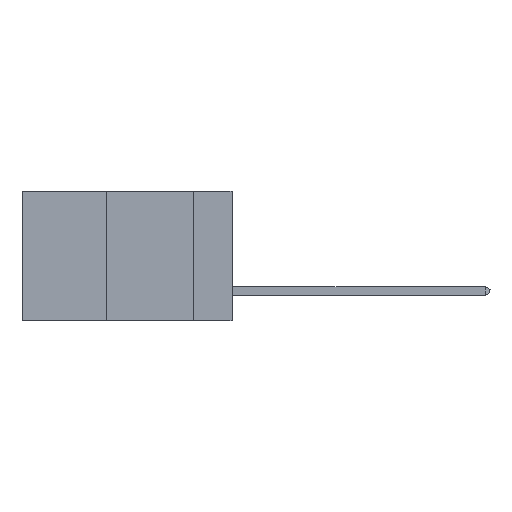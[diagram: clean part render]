
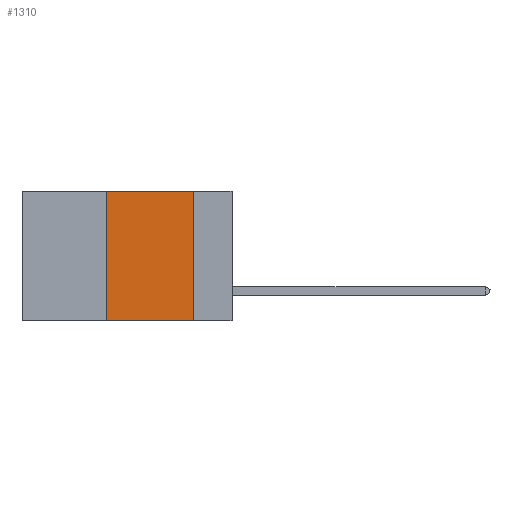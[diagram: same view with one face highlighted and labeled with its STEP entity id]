
A CAD part, left-side view. The second image highlights one B-rep face of the part: STEP entity #1310.
In plain terms, the highlighted planar face has unit normal (-1, 0, 0).
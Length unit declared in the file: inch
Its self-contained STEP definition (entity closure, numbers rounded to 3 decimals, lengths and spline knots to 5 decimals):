
#838 = ORIENTED_EDGE ( 'NONE', *, *, #8787, .F. ) ;
#1310 = ADVANCED_FACE ( 'NONE', ( #13364 ), #34710, .F. ) ;
#1548 = VECTOR ( 'NONE', #7268, 39.37008 ) ;
#2226 = DIRECTION ( 'NONE',  ( 0., 0., -1. ) ) ;
#2724 = ORIENTED_EDGE ( 'NONE', *, *, #13543, .F. ) ;
#6055 = EDGE_CURVE ( 'NONE', #22700, #18004, #16288, .T. ) ;
#7268 = DIRECTION ( 'NONE',  ( 0., 0., 1. ) ) ;
#8787 = EDGE_CURVE ( 'NONE', #15498, #22700, #21053, .T. ) ;
#9929 = CARTESIAN_POINT ( 'NONE',  ( 0., 0.36, 0. ) ) ;
#10812 = VECTOR ( 'NONE', #12277, 39.37008 ) ;
#11477 = ORIENTED_EDGE ( 'NONE', *, *, #6055, .F. ) ;
#11545 = CARTESIAN_POINT ( 'NONE',  ( 0., 0.11, 0. ) ) ;
#11572 = CARTESIAN_POINT ( 'NONE',  ( 0., 0.11, -0.37 ) ) ;
#12277 = DIRECTION ( 'NONE',  ( 0., -1., 0. ) ) ;
#13058 = EDGE_CURVE ( 'NONE', #13411, #18004, #17868, .T. ) ;
#13364 = FACE_OUTER_BOUND ( 'NONE', #16948, .T. ) ;
#13411 = VERTEX_POINT ( 'NONE', #15397 ) ;
#13543 = EDGE_CURVE ( 'NONE', #13411, #15498, #41147, .T. ) ;
#15269 = DIRECTION ( 'NONE',  ( 0., 0., -1. ) ) ;
#15397 = CARTESIAN_POINT ( 'NONE',  ( 0., 0.36, -0.37 ) ) ;
#15498 = VERTEX_POINT ( 'NONE', #9929 ) ;
#16288 = LINE ( 'NONE', #11545, #22893 ) ;
#16948 = EDGE_LOOP ( 'NONE', ( #11477, #838, #2724, #37770 ) ) ;
#17868 = LINE ( 'NONE', #36186, #40135 ) ;
#18004 = VERTEX_POINT ( 'NONE', #11572 ) ;
#21053 = LINE ( 'NONE', #32386, #10812 ) ;
#22700 = VERTEX_POINT ( 'NONE', #23381 ) ;
#22893 = VECTOR ( 'NONE', #15269, 39.37008 ) ;
#23381 = CARTESIAN_POINT ( 'NONE',  ( 0., 0.11, 0. ) ) ;
#23920 = DIRECTION ( 'NONE',  ( 0., -1., 0. ) ) ;
#25184 = DIRECTION ( 'NONE',  ( 1., 0., 0. ) ) ;
#29550 = CARTESIAN_POINT ( 'NONE',  ( 0., 0.36, 0. ) ) ;
#32386 = CARTESIAN_POINT ( 'NONE',  ( 0., 0.6, 0. ) ) ;
#34710 = PLANE ( 'NONE',  #41684 ) ;
#36186 = CARTESIAN_POINT ( 'NONE',  ( 0., 0.6, -0.37 ) ) ;
#37770 = ORIENTED_EDGE ( 'NONE', *, *, #13058, .T. ) ;
#38151 = CARTESIAN_POINT ( 'NONE',  ( 0., 0.6, 0. ) ) ;
#40135 = VECTOR ( 'NONE', #23920, 39.37008 ) ;
#41147 = LINE ( 'NONE', #29550, #1548 ) ;
#41684 = AXIS2_PLACEMENT_3D ( 'NONE', #38151, #25184, #2226 ) ;
